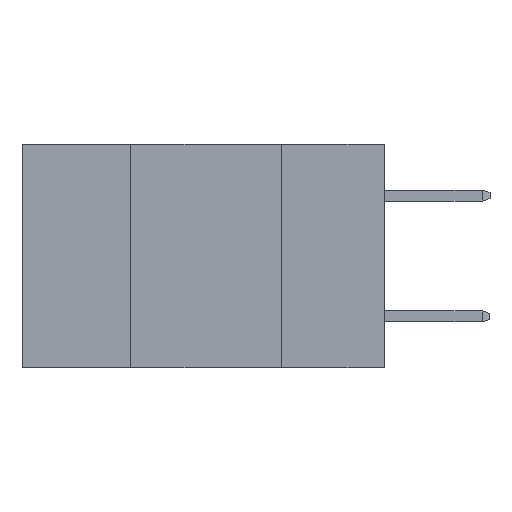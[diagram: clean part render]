
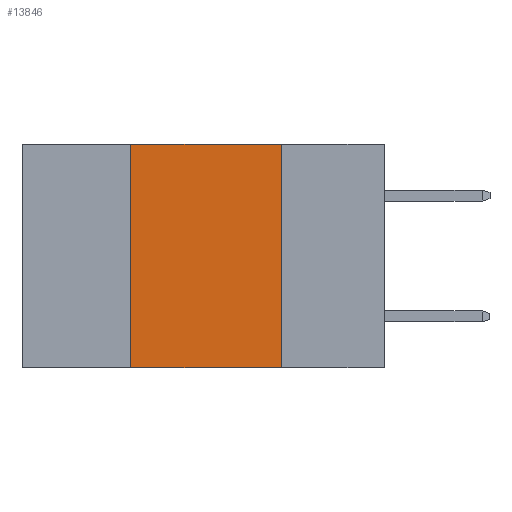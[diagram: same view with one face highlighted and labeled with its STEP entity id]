
A CAD part, left-side view. The second image highlights one B-rep face of the part: STEP entity #13846.
In plain terms, the highlighted planar face has unit normal (-1, 0, 0).
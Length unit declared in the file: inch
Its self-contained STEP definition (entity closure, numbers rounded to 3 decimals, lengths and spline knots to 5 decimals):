
#295 = EDGE_LOOP ( 'NONE', ( #629, #4295, #12021, #9654 ) ) ;
#321 = CARTESIAN_POINT ( 'NONE',  ( 0., 0.42, -0.37 ) ) ;
#609 = DIRECTION ( 'NONE',  ( 0., 0., -1. ) ) ;
#629 = ORIENTED_EDGE ( 'NONE', *, *, #13251, .F. ) ;
#900 = VECTOR ( 'NONE', #15800, 39.37008 ) ;
#996 = VERTEX_POINT ( 'NONE', #321 ) ;
#1302 = EDGE_CURVE ( 'NONE', #9697, #3698, #14414, .T. ) ;
#1975 = AXIS2_PLACEMENT_3D ( 'NONE', #7967, #9482, #609 ) ;
#2387 = CARTESIAN_POINT ( 'NONE',  ( 0., 0.6, -0.37 ) ) ;
#3124 = VECTOR ( 'NONE', #5065, 39.37008 ) ;
#3437 = PLANE ( 'NONE',  #1975 ) ;
#3698 = VERTEX_POINT ( 'NONE', #6613 ) ;
#4295 = ORIENTED_EDGE ( 'NONE', *, *, #1302, .F. ) ;
#5065 = DIRECTION ( 'NONE',  ( 0., 0., -1. ) ) ;
#6481 = VECTOR ( 'NONE', #16425, 39.37008 ) ;
#6613 = CARTESIAN_POINT ( 'NONE',  ( 0., 0.17, 0. ) ) ;
#7967 = CARTESIAN_POINT ( 'NONE',  ( 0., 0.6, 0. ) ) ;
#7992 = CARTESIAN_POINT ( 'NONE',  ( 0., 0.17, 0. ) ) ;
#7996 = CARTESIAN_POINT ( 'NONE',  ( 0., 0.17, -0.37 ) ) ;
#9482 = DIRECTION ( 'NONE',  ( 1., 0., 0. ) ) ;
#9654 = ORIENTED_EDGE ( 'NONE', *, *, #17090, .T. ) ;
#9697 = VERTEX_POINT ( 'NONE', #12298 ) ;
#11046 = LINE ( 'NONE', #7992, #3124 ) ;
#11072 = VECTOR ( 'NONE', #15964, 39.37008 ) ;
#11109 = VERTEX_POINT ( 'NONE', #7996 ) ;
#11467 = CARTESIAN_POINT ( 'NONE',  ( 0., 0.42, 0. ) ) ;
#12021 = ORIENTED_EDGE ( 'NONE', *, *, #19148, .F. ) ;
#12298 = CARTESIAN_POINT ( 'NONE',  ( 0., 0.42, 0. ) ) ;
#13251 = EDGE_CURVE ( 'NONE', #3698, #11109, #11046, .T. ) ;
#13846 = ADVANCED_FACE ( 'NONE', ( #15680 ), #3437, .F. ) ;
#14239 = CARTESIAN_POINT ( 'NONE',  ( 0., 0.6, 0. ) ) ;
#14414 = LINE ( 'NONE', #14239, #6481 ) ;
#15680 = FACE_OUTER_BOUND ( 'NONE', #295, .T. ) ;
#15800 = DIRECTION ( 'NONE',  ( 0., -1., 0. ) ) ;
#15964 = DIRECTION ( 'NONE',  ( 0., 0., 1. ) ) ;
#16176 = LINE ( 'NONE', #11467, #11072 ) ;
#16425 = DIRECTION ( 'NONE',  ( 0., -1., 0. ) ) ;
#16714 = LINE ( 'NONE', #2387, #900 ) ;
#17090 = EDGE_CURVE ( 'NONE', #996, #11109, #16714, .T. ) ;
#19148 = EDGE_CURVE ( 'NONE', #996, #9697, #16176, .T. ) ;
